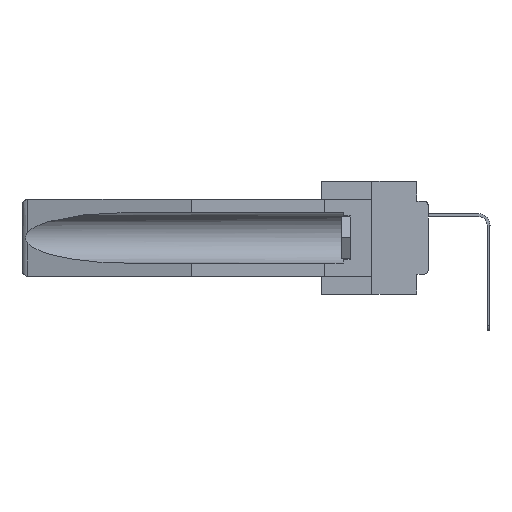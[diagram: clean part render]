
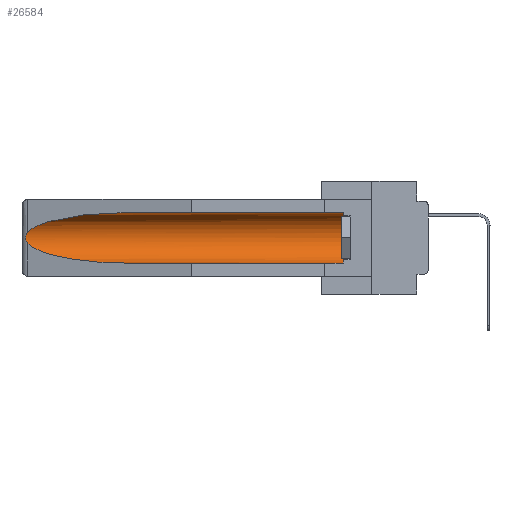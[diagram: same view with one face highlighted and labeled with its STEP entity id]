
A CAD part, left-side view. The second image highlights one B-rep face of the part: STEP entity #26584.
In plain terms, the highlighted cylindrical face has radius 2.857 mm (diameter 5.715 mm), a partial arc.
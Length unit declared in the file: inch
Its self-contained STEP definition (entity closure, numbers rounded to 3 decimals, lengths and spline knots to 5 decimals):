
#1993 = ORIENTED_EDGE ( 'NONE', *, *, #16702, .T. ) ;
#3339 = CARTESIAN_POINT ( 'NONE',  ( 0.155, 1.07973, -0.059 ) ) ;
#3644 = CARTESIAN_POINT ( 'NONE',  ( 0.155, 0.126, -0.059 ) ) ;
#3883 = B_SPLINE_CURVE_WITH_KNOTS ( 'NONE', 3,
 ( #4600, #6862, #26698, #31527, #19488, #24134, #26589, #16892, #11816, #4713 ),
 .UNSPECIFIED., .F., .F.,
 ( 4, 2, 2, 2, 4 ),
 ( 0., 0.00029, 0.00058, 0.00087, 0.00117 ),
 .UNSPECIFIED. ) ;
#4600 = CARTESIAN_POINT ( 'NONE',  ( 0.26537, 1.52718, -0.14972 ) ) ;
#4713 = CARTESIAN_POINT ( 'NONE',  ( 0.26537, 1.52718, -0.19328 ) ) ;
#4738 = ORIENTED_EDGE ( 'NONE', *, *, #5423, .F. ) ;
#4932 = CARTESIAN_POINT ( 'NONE',  ( 0.26537, 1.52718, -0.19328 ) ) ;
#5244 = CARTESIAN_POINT ( 'NONE',  ( 0.155, 1.07973, -0.284 ) ) ;
#5423 = EDGE_CURVE ( 'NONE', #12766, #17489, #26448, .T. ) ;
#5488 = DIRECTION ( 'NONE',  ( 0., 1., 0. ) ) ;
#5721 = ORIENTED_EDGE ( 'NONE', *, *, #16604, .T. ) ;
#5801 = EDGE_CURVE ( 'NONE', #8528, #29719, #22138, .T. ) ;
#6085 = EDGE_CURVE ( 'NONE', #12766, #7636, #16759, .T. ) ;
#6862 = CARTESIAN_POINT ( 'NONE',  ( 0.26597, 1.52961, -0.15275 ) ) ;
#7282 = CARTESIAN_POINT ( 'NONE',  ( 0.21114, 1.30732, -0.284 ) ) ;
#7513 = DIRECTION ( 'NONE',  ( 0., 0., 1. ) ) ;
#7572 = AXIS2_PLACEMENT_3D ( 'NONE', #22367, #5488, #12502 ) ;
#7636 = VERTEX_POINT ( 'NONE', #3644 ) ;
#7965 = FACE_OUTER_BOUND ( 'NONE', #11990, .T. ) ;
#8528 = VERTEX_POINT ( 'NONE', #9721 ) ;
#9721 = CARTESIAN_POINT ( 'NONE',  ( 0.155, 1.07973, -0.059 ) ) ;
#9927 = CARTESIAN_POINT ( 'NONE',  ( 0.26537, 1.52718, -0.19328 ) ) ;
#11608 = VERTEX_POINT ( 'NONE', #9927 ) ;
#11816 = CARTESIAN_POINT ( 'NONE',  ( 0.26597, 1.5296, -0.19026 ) ) ;
#11939 = DIRECTION ( 'NONE',  ( 0., -1., 0. ) ) ;
#11990 = EDGE_LOOP ( 'NONE', ( #14117, #5721, #1993, #4738, #14454, #29675 ) ) ;
#12502 = DIRECTION ( 'NONE',  ( 0., 0., 1. ) ) ;
#12668 = CARTESIAN_POINT ( 'NONE',  ( 0.25451, 1.48313, -0.24835 ) ) ;
#12766 = VERTEX_POINT ( 'NONE', #24929 ) ;
#14117 = ORIENTED_EDGE ( 'NONE', *, *, #5801, .T. ) ;
#14454 = ORIENTED_EDGE ( 'NONE', *, *, #6085, .T. ) ;
#15377 = CARTESIAN_POINT ( 'NONE',  ( 0.155, 1.07973, -0.284 ) ) ;
#15841 = CARTESIAN_POINT ( 'NONE',  ( 0.155, -0.30754, -0.059 ) ) ;
#16604 = EDGE_CURVE ( 'NONE', #29719, #11608, #3883, .T. ) ;
#16702 = EDGE_CURVE ( 'NONE', #11608, #17489, #29177, .T. ) ;
#16759 = CIRCLE ( 'NONE', #25096, 0.1125 ) ;
#16892 = CARTESIAN_POINT ( 'NONE',  ( 0.26655, 1.53094, -0.18657 ) ) ;
#17489 = VERTEX_POINT ( 'NONE', #15377 ) ;
#17618 = CYLINDRICAL_SURFACE ( 'NONE', #7572, 0.1125 ) ;
#19233 = VECTOR ( 'NONE', #25679, 39.37008 ) ;
#19488 = CARTESIAN_POINT ( 'NONE',  ( 0.2675, 1.53308, -0.16763 ) ) ;
#19607 = CARTESIAN_POINT ( 'NONE',  ( 0.155, 0.126, -0.1715 ) ) ;
#20294 = CARTESIAN_POINT ( 'NONE',  ( 0.26537, 1.52718, -0.14972 ) ) ;
#20811 = LINE ( 'NONE', #15841, #19233 ) ;
#22136 = CARTESIAN_POINT ( 'NONE',  ( 0.155, -0.30754, -0.284 ) ) ;
#22138 =( BOUNDED_CURVE ( )  B_SPLINE_CURVE ( 3, ( #3339, #22994, #27711, #20294 ),
 .UNSPECIFIED., .F., .F. ) 
 B_SPLINE_CURVE_WITH_KNOTS ( ( 4, 4 ),
 ( 4.71239, 6.08839 ),
 .UNSPECIFIED. ) 
 CURVE ( )  GEOMETRIC_REPRESENTATION_ITEM ( )  RATIONAL_B_SPLINE_CURVE ( ( 1., 0.848, 0.848, 1. ) ) 
 REPRESENTATION_ITEM ( '' )  );
#22367 = CARTESIAN_POINT ( 'NONE',  ( 0.155, -0.30754, -0.1715 ) ) ;
#22994 = CARTESIAN_POINT ( 'NONE',  ( 0.21114, 1.30732, -0.059 ) ) ;
#23374 = EDGE_CURVE ( 'NONE', #7636, #8528, #20811, .T. ) ;
#24134 = CARTESIAN_POINT ( 'NONE',  ( 0.2675, 1.53308, -0.17534 ) ) ;
#24249 = CARTESIAN_POINT ( 'NONE',  ( 0.26537, 1.52718, -0.14972 ) ) ;
#24929 = CARTESIAN_POINT ( 'NONE',  ( 0.155, 0.126, -0.284 ) ) ;
#25096 = AXIS2_PLACEMENT_3D ( 'NONE', #19607, #11939, #7513 ) ;
#25316 = VECTOR ( 'NONE', #29505, 39.37008 ) ;
#25679 = DIRECTION ( 'NONE',  ( 0., 1., 0. ) ) ;
#26448 = LINE ( 'NONE', #22136, #25316 ) ;
#26584 = ADVANCED_FACE ( 'NONE', ( #7965 ), #17618, .F. ) ;
#26589 = CARTESIAN_POINT ( 'NONE',  ( 0.2673, 1.53269, -0.17917 ) ) ;
#26698 = CARTESIAN_POINT ( 'NONE',  ( 0.26654, 1.53092, -0.15636 ) ) ;
#27711 = CARTESIAN_POINT ( 'NONE',  ( 0.25451, 1.48313, -0.09465 ) ) ;
#29177 =( BOUNDED_CURVE ( )  B_SPLINE_CURVE ( 3, ( #4932, #12668, #7282, #5244 ),
 .UNSPECIFIED., .F., .F. ) 
 B_SPLINE_CURVE_WITH_KNOTS ( ( 4, 4 ),
 ( 0.1948, 1.5708 ),
 .UNSPECIFIED. ) 
 CURVE ( )  GEOMETRIC_REPRESENTATION_ITEM ( )  RATIONAL_B_SPLINE_CURVE ( ( 1., 0.848, 0.848, 1. ) ) 
 REPRESENTATION_ITEM ( '' )  );
#29505 = DIRECTION ( 'NONE',  ( 0., 1., 0. ) ) ;
#29675 = ORIENTED_EDGE ( 'NONE', *, *, #23374, .T. ) ;
#29719 = VERTEX_POINT ( 'NONE', #24249 ) ;
#31527 = CARTESIAN_POINT ( 'NONE',  ( 0.2673, 1.5327, -0.16383 ) ) ;
